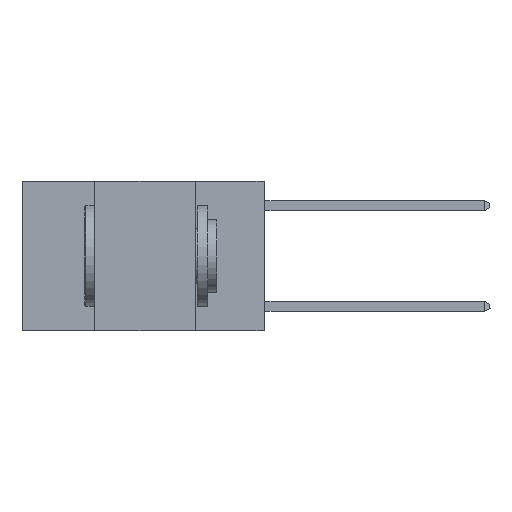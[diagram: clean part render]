
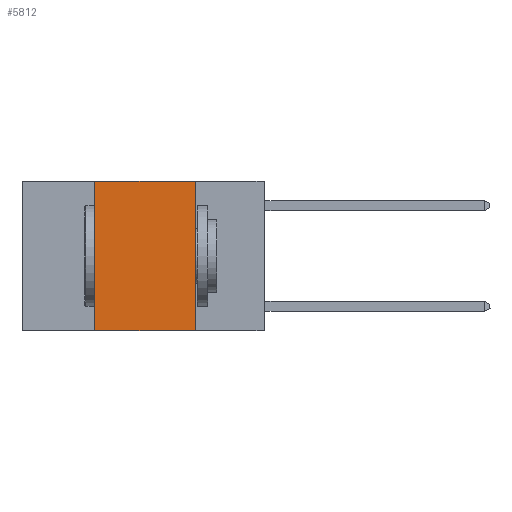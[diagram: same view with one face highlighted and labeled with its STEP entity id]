
A CAD part, left-side view. The second image highlights one B-rep face of the part: STEP entity #5812.
In plain terms, the highlighted planar face has unit normal (-1, 0, 0).
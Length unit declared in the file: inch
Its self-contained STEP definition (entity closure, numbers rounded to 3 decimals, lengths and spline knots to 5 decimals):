
#18 = LINE ( 'NONE', #5496, #2426 ) ;
#247 = CARTESIAN_POINT ( 'NONE',  ( 0., 0.42, -0.37 ) ) ;
#1080 = VERTEX_POINT ( 'NONE', #3102 ) ;
#1108 = VERTEX_POINT ( 'NONE', #11014 ) ;
#1629 = VECTOR ( 'NONE', #11279, 39.37008 ) ;
#1837 = PLANE ( 'NONE',  #10880 ) ;
#1906 = CARTESIAN_POINT ( 'NONE',  ( 0., 0.6, 0. ) ) ;
#2373 = EDGE_CURVE ( 'NONE', #2618, #1108, #18, .T. ) ;
#2426 = VECTOR ( 'NONE', #10849, 39.37008 ) ;
#2618 = VERTEX_POINT ( 'NONE', #247 ) ;
#3102 = CARTESIAN_POINT ( 'NONE',  ( 0., 0.42, 0. ) ) ;
#4395 = DIRECTION ( 'NONE',  ( 0., 0., 1. ) ) ;
#4622 = EDGE_CURVE ( 'NONE', #11834, #1108, #7387, .T. ) ;
#5029 = FACE_OUTER_BOUND ( 'NONE', #11605, .T. ) ;
#5366 = CARTESIAN_POINT ( 'NONE',  ( 0., 0.42, 0. ) ) ;
#5496 = CARTESIAN_POINT ( 'NONE',  ( 0., 0.6, -0.37 ) ) ;
#5696 = DIRECTION ( 'NONE',  ( 1., 0., 0. ) ) ;
#5812 = ADVANCED_FACE ( 'NONE', ( #5029 ), #1837, .F. ) ;
#5963 = DIRECTION ( 'NONE',  ( 0., 0., -1. ) ) ;
#6431 = LINE ( 'NONE', #1906, #1629 ) ;
#7387 = LINE ( 'NONE', #9637, #12123 ) ;
#8941 = EDGE_CURVE ( 'NONE', #1080, #11834, #6431, .T. ) ;
#9103 = CARTESIAN_POINT ( 'NONE',  ( 0., 0.17, 0. ) ) ;
#9637 = CARTESIAN_POINT ( 'NONE',  ( 0., 0.17, 0. ) ) ;
#10246 = ORIENTED_EDGE ( 'NONE', *, *, #2373, .T. ) ;
#10745 = ORIENTED_EDGE ( 'NONE', *, *, #8941, .F. ) ;
#10849 = DIRECTION ( 'NONE',  ( 0., -1., 0. ) ) ;
#10880 = AXIS2_PLACEMENT_3D ( 'NONE', #11304, #5696, #12269 ) ;
#10891 = ORIENTED_EDGE ( 'NONE', *, *, #4622, .F. ) ;
#11014 = CARTESIAN_POINT ( 'NONE',  ( 0., 0.17, -0.37 ) ) ;
#11279 = DIRECTION ( 'NONE',  ( 0., -1., 0. ) ) ;
#11304 = CARTESIAN_POINT ( 'NONE',  ( 0., 0.6, 0. ) ) ;
#11305 = ORIENTED_EDGE ( 'NONE', *, *, #11807, .F. ) ;
#11605 = EDGE_LOOP ( 'NONE', ( #10891, #10745, #11305, #10246 ) ) ;
#11703 = LINE ( 'NONE', #5366, #12017 ) ;
#11807 = EDGE_CURVE ( 'NONE', #2618, #1080, #11703, .T. ) ;
#11834 = VERTEX_POINT ( 'NONE', #9103 ) ;
#12017 = VECTOR ( 'NONE', #4395, 39.37008 ) ;
#12123 = VECTOR ( 'NONE', #5963, 39.37008 ) ;
#12269 = DIRECTION ( 'NONE',  ( 0., 0., -1. ) ) ;
